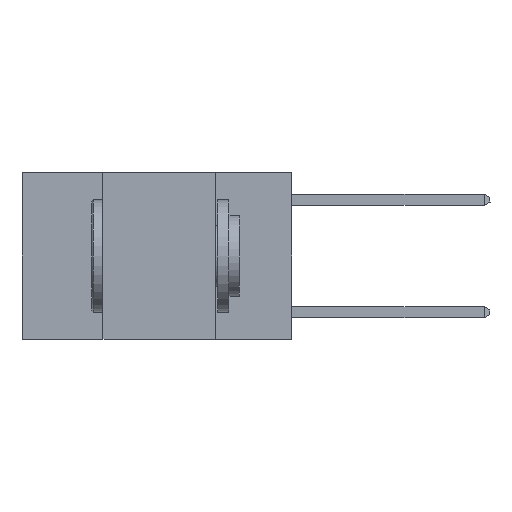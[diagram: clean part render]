
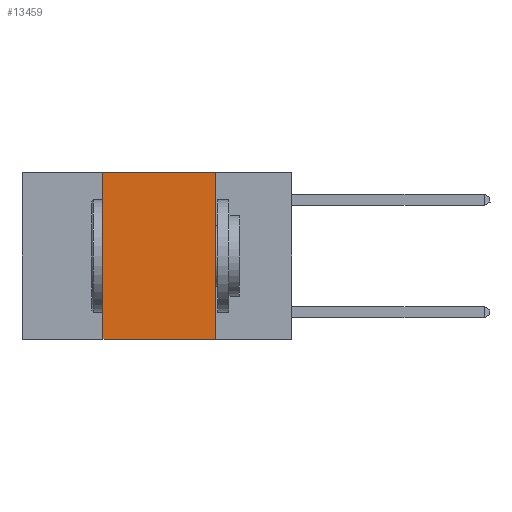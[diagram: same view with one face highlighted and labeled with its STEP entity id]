
A CAD part, left-side view. The second image highlights one B-rep face of the part: STEP entity #13459.
In plain terms, the highlighted planar face has unit normal (-1, 0, 0).
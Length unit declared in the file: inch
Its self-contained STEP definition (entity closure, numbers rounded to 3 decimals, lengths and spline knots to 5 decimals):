
#67 = DIRECTION ( 'NONE',  ( 1., 0., 0. ) ) ;
#1766 = CARTESIAN_POINT ( 'NONE',  ( 0., 0.17, 0. ) ) ;
#2110 = CARTESIAN_POINT ( 'NONE',  ( 0., 0.42, 0. ) ) ;
#2800 = CARTESIAN_POINT ( 'NONE',  ( 0., 0.17, 0. ) ) ;
#3570 = LINE ( 'NONE', #4049, #8529 ) ;
#4049 = CARTESIAN_POINT ( 'NONE',  ( 0., 0.6, -0.37 ) ) ;
#4922 = ORIENTED_EDGE ( 'NONE', *, *, #15001, .F. ) ;
#5336 = EDGE_CURVE ( 'NONE', #18669, #9883, #5957, .T. ) ;
#5566 = FACE_OUTER_BOUND ( 'NONE', #11385, .T. ) ;
#5957 = LINE ( 'NONE', #16523, #15104 ) ;
#6697 = VERTEX_POINT ( 'NONE', #8619 ) ;
#7527 = ORIENTED_EDGE ( 'NONE', *, *, #12582, .F. ) ;
#7646 = EDGE_CURVE ( 'NONE', #6697, #14880, #3570, .T. ) ;
#8527 = CARTESIAN_POINT ( 'NONE',  ( 0., 0.42, 0. ) ) ;
#8529 = VECTOR ( 'NONE', #15054, 39.37008 ) ;
#8619 = CARTESIAN_POINT ( 'NONE',  ( 0., 0.42, -0.37 ) ) ;
#9348 = PLANE ( 'NONE',  #13130 ) ;
#9883 = VERTEX_POINT ( 'NONE', #2800 ) ;
#11385 = EDGE_LOOP ( 'NONE', ( #4922, #21881, #7527, #14254 ) ) ;
#12582 = EDGE_CURVE ( 'NONE', #6697, #18669, #22404, .T. ) ;
#13065 = DIRECTION ( 'NONE',  ( 0., 0., -1. ) ) ;
#13130 = AXIS2_PLACEMENT_3D ( 'NONE', #21963, #67, #13065 ) ;
#13459 = ADVANCED_FACE ( 'NONE', ( #5566 ), #9348, .F. ) ;
#14254 = ORIENTED_EDGE ( 'NONE', *, *, #7646, .T. ) ;
#14670 = DIRECTION ( 'NONE',  ( 0., 0., -1. ) ) ;
#14880 = VERTEX_POINT ( 'NONE', #16179 ) ;
#15001 = EDGE_CURVE ( 'NONE', #9883, #14880, #16061, .T. ) ;
#15054 = DIRECTION ( 'NONE',  ( 0., -1., 0. ) ) ;
#15104 = VECTOR ( 'NONE', #18306, 39.37008 ) ;
#16061 = LINE ( 'NONE', #1766, #21363 ) ;
#16179 = CARTESIAN_POINT ( 'NONE',  ( 0., 0.17, -0.37 ) ) ;
#16523 = CARTESIAN_POINT ( 'NONE',  ( 0., 0.6, 0. ) ) ;
#17690 = VECTOR ( 'NONE', #19470, 39.37008 ) ;
#18306 = DIRECTION ( 'NONE',  ( 0., -1., 0. ) ) ;
#18669 = VERTEX_POINT ( 'NONE', #2110 ) ;
#19470 = DIRECTION ( 'NONE',  ( 0., 0., 1. ) ) ;
#21363 = VECTOR ( 'NONE', #14670, 39.37008 ) ;
#21881 = ORIENTED_EDGE ( 'NONE', *, *, #5336, .F. ) ;
#21963 = CARTESIAN_POINT ( 'NONE',  ( 0., 0.6, 0. ) ) ;
#22404 = LINE ( 'NONE', #8527, #17690 ) ;
